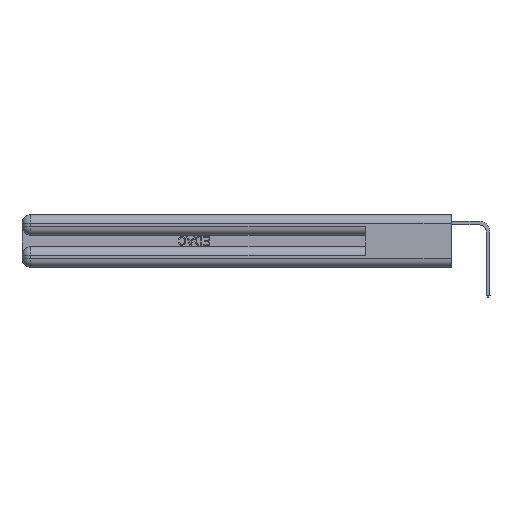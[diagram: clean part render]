
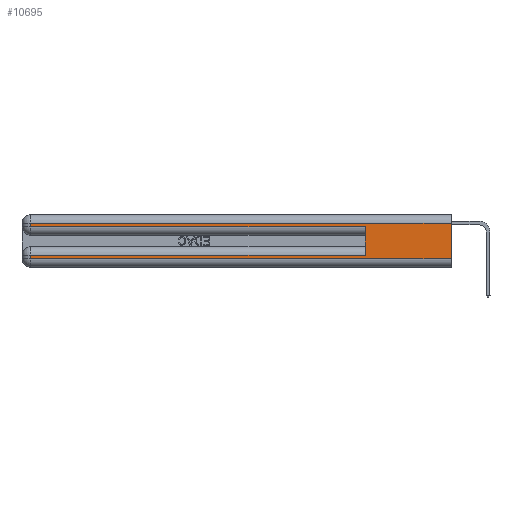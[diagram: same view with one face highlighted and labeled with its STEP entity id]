
A CAD part, left-side view. The second image highlights one B-rep face of the part: STEP entity #10695.
In plain terms, the highlighted planar face has unit normal (-1, 0, 0).
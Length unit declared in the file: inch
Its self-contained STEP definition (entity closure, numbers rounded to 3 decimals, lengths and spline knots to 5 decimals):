
#116 = LINE ( 'NONE', #10856, #31391 ) ;
#849 = CARTESIAN_POINT ( 'NONE',  ( 0., 0., 0.37 ) ) ;
#933 = VERTEX_POINT ( 'NONE', #23036 ) ;
#1907 = EDGE_CURVE ( 'NONE', #933, #32392, #31920, .T. ) ;
#1972 = CARTESIAN_POINT ( 'NONE',  ( 0., 0., 0.37 ) ) ;
#2373 = CARTESIAN_POINT ( 'NONE',  ( 0., 0.6, 0.145 ) ) ;
#2552 = VECTOR ( 'NONE', #33552, 39.37008 ) ;
#2606 = VERTEX_POINT ( 'NONE', #15827 ) ;
#3322 = VECTOR ( 'NONE', #13933, 39.37008 ) ;
#3541 = VERTEX_POINT ( 'NONE', #31263 ) ;
#4405 = DIRECTION ( 'NONE',  ( 0., 0., -1. ) ) ;
#5353 = EDGE_CURVE ( 'NONE', #933, #10085, #20389, .T. ) ;
#6140 = ORIENTED_EDGE ( 'NONE', *, *, #13126, .F. ) ;
#6619 = CARTESIAN_POINT ( 'NONE',  ( 0., 2.94, 0.37 ) ) ;
#7141 = CARTESIAN_POINT ( 'NONE',  ( 0., 0., 0.06 ) ) ;
#8129 = CARTESIAN_POINT ( 'NONE',  ( 0., 2.94, 0.285 ) ) ;
#8410 = ORIENTED_EDGE ( 'NONE', *, *, #1907, .T. ) ;
#8849 = CARTESIAN_POINT ( 'NONE',  ( 0., 2.94, 0.085 ) ) ;
#8953 = ORIENTED_EDGE ( 'NONE', *, *, #20712, .T. ) ;
#9265 = AXIS2_PLACEMENT_3D ( 'NONE', #849, #29490, #27275 ) ;
#9602 = EDGE_CURVE ( 'NONE', #3541, #10085, #28280, .T. ) ;
#10085 = VERTEX_POINT ( 'NONE', #15612 ) ;
#10212 = DIRECTION ( 'NONE',  ( 0., 0., 1. ) ) ;
#10695 = ADVANCED_FACE ( 'NONE', ( #14322 ), #16705, .F. ) ;
#10856 = CARTESIAN_POINT ( 'NONE',  ( 0., 0., 0.085 ) ) ;
#11404 = VECTOR ( 'NONE', #17543, 39.37008 ) ;
#11550 = VECTOR ( 'NONE', #10212, 39.37008 ) ;
#11785 = CARTESIAN_POINT ( 'NONE',  ( 0., 2.94, 0.31 ) ) ;
#11877 = VECTOR ( 'NONE', #26634, 39.37008 ) ;
#13126 = EDGE_CURVE ( 'NONE', #20487, #2606, #15330, .T. ) ;
#13933 = DIRECTION ( 'NONE',  ( 0., -1., 0. ) ) ;
#14322 = FACE_OUTER_BOUND ( 'NONE', #33062, .T. ) ;
#15330 = LINE ( 'NONE', #2373, #11550 ) ;
#15612 = CARTESIAN_POINT ( 'NONE',  ( 0., 0., 0.06 ) ) ;
#15632 = LINE ( 'NONE', #17860, #2552 ) ;
#15640 = VECTOR ( 'NONE', #17667, 39.37008 ) ;
#15827 = CARTESIAN_POINT ( 'NONE',  ( 0., 0.6, 0.285 ) ) ;
#16705 = PLANE ( 'NONE',  #9265 ) ;
#17194 = LINE ( 'NONE', #6619, #18449 ) ;
#17543 = DIRECTION ( 'NONE',  ( 0., -1., 0. ) ) ;
#17667 = DIRECTION ( 'NONE',  ( 0., 0., -1. ) ) ;
#17860 = CARTESIAN_POINT ( 'NONE',  ( 0., 2.94, 0.37 ) ) ;
#18275 = EDGE_CURVE ( 'NONE', #20487, #26243, #116, .T. ) ;
#18449 = VECTOR ( 'NONE', #4405, 39.37008 ) ;
#18807 = CARTESIAN_POINT ( 'NONE',  ( 0., 0., 0.31 ) ) ;
#20153 = ORIENTED_EDGE ( 'NONE', *, *, #5353, .F. ) ;
#20389 = LINE ( 'NONE', #1972, #15640 ) ;
#20485 = ORIENTED_EDGE ( 'NONE', *, *, #26705, .T. ) ;
#20487 = VERTEX_POINT ( 'NONE', #32029 ) ;
#20712 = EDGE_CURVE ( 'NONE', #32392, #22216, #15632, .T. ) ;
#21417 = DIRECTION ( 'NONE',  ( 0., 1., 0. ) ) ;
#22216 = VERTEX_POINT ( 'NONE', #8129 ) ;
#22875 = ORIENTED_EDGE ( 'NONE', *, *, #23014, .T. ) ;
#23014 = EDGE_CURVE ( 'NONE', #26243, #3541, #17194, .T. ) ;
#23015 = ORIENTED_EDGE ( 'NONE', *, *, #18275, .T. ) ;
#23036 = CARTESIAN_POINT ( 'NONE',  ( 0., 0., 0.31 ) ) ;
#24497 = LINE ( 'NONE', #27042, #3322 ) ;
#26243 = VERTEX_POINT ( 'NONE', #8849 ) ;
#26634 = DIRECTION ( 'NONE',  ( 0., 1., 0. ) ) ;
#26705 = EDGE_CURVE ( 'NONE', #22216, #2606, #24497, .T. ) ;
#27042 = CARTESIAN_POINT ( 'NONE',  ( 0., 0., 0.285 ) ) ;
#27275 = DIRECTION ( 'NONE',  ( 0., 0., -1. ) ) ;
#28280 = LINE ( 'NONE', #7141, #11404 ) ;
#29490 = DIRECTION ( 'NONE',  ( 1., 0., 0. ) ) ;
#30852 = ORIENTED_EDGE ( 'NONE', *, *, #9602, .T. ) ;
#31263 = CARTESIAN_POINT ( 'NONE',  ( 0., 2.94, 0.06 ) ) ;
#31391 = VECTOR ( 'NONE', #21417, 39.37008 ) ;
#31920 = LINE ( 'NONE', #18807, #11877 ) ;
#32029 = CARTESIAN_POINT ( 'NONE',  ( 0., 0.6, 0.085 ) ) ;
#32392 = VERTEX_POINT ( 'NONE', #11785 ) ;
#33062 = EDGE_LOOP ( 'NONE', ( #20153, #8410, #8953, #20485, #6140, #23015, #22875, #30852 ) ) ;
#33552 = DIRECTION ( 'NONE',  ( 0., 0., -1. ) ) ;
